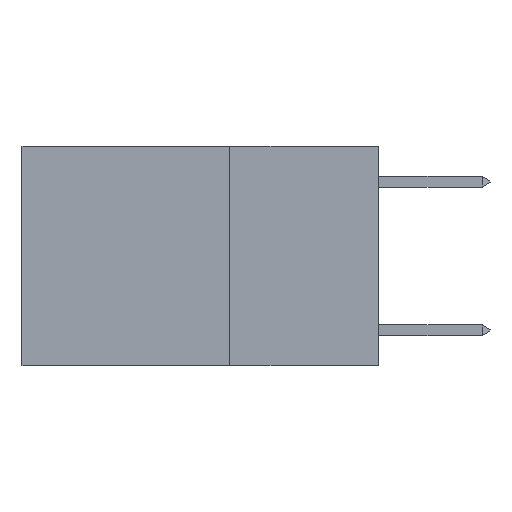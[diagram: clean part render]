
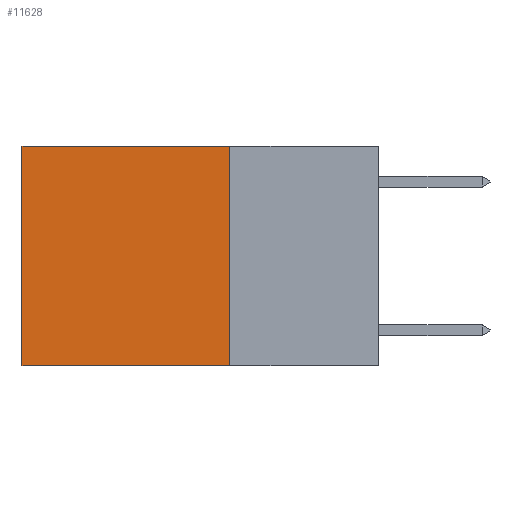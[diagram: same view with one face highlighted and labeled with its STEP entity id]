
A CAD part, left-side view. The second image highlights one B-rep face of the part: STEP entity #11628.
In plain terms, the highlighted planar face has unit normal (-1, 0, 0).
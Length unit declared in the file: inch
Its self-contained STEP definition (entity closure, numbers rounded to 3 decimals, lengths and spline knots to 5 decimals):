
#13 = CARTESIAN_POINT ( 'NONE',  ( 0.2625, 0.25, -0.37 ) ) ;
#211 = DIRECTION ( 'NONE',  ( 0., 0., -1. ) ) ;
#406 = DIRECTION ( 'NONE',  ( 1., 0., 0. ) ) ;
#1454 = DIRECTION ( 'NONE',  ( 0., 0., -1. ) ) ;
#2132 = ORIENTED_EDGE ( 'NONE', *, *, #9525, .F. ) ;
#2313 = CARTESIAN_POINT ( 'NONE',  ( 0.2625, 0.25, 0. ) ) ;
#2341 = CARTESIAN_POINT ( 'NONE',  ( 0.2625, 0.6, 0. ) ) ;
#3111 = EDGE_LOOP ( 'NONE', ( #7426, #9979, #2132, #9470 ) ) ;
#3143 = CARTESIAN_POINT ( 'NONE',  ( 0.2625, 0.25, 0. ) ) ;
#3300 = VERTEX_POINT ( 'NONE', #10219 ) ;
#3956 = LINE ( 'NONE', #13, #11379 ) ;
#4153 = LINE ( 'NONE', #3143, #11123 ) ;
#4418 = EDGE_CURVE ( 'NONE', #9586, #8267, #7765, .T. ) ;
#4705 = DIRECTION ( 'NONE',  ( 0., 0., -1. ) ) ;
#4857 = AXIS2_PLACEMENT_3D ( 'NONE', #2313, #406, #211 ) ;
#5376 = LINE ( 'NONE', #6614, #8324 ) ;
#5546 = PLANE ( 'NONE',  #4857 ) ;
#5997 = CARTESIAN_POINT ( 'NONE',  ( 0.2625, 0.6, -0.37 ) ) ;
#6614 = CARTESIAN_POINT ( 'NONE',  ( 0.2625, 0.25, 0. ) ) ;
#6640 = EDGE_CURVE ( 'NONE', #3300, #9586, #4153, .T. ) ;
#7263 = DIRECTION ( 'NONE',  ( 0., 1., 0. ) ) ;
#7426 = ORIENTED_EDGE ( 'NONE', *, *, #4418, .T. ) ;
#7758 = VECTOR ( 'NONE', #4705, 39.37008 ) ;
#7765 = LINE ( 'NONE', #11892, #7758 ) ;
#8093 = DIRECTION ( 'NONE',  ( 0., 1., 0. ) ) ;
#8267 = VERTEX_POINT ( 'NONE', #5997 ) ;
#8324 = VECTOR ( 'NONE', #1454, 39.37008 ) ;
#9436 = CARTESIAN_POINT ( 'NONE',  ( 0.2625, 0.25, -0.37 ) ) ;
#9470 = ORIENTED_EDGE ( 'NONE', *, *, #6640, .T. ) ;
#9525 = EDGE_CURVE ( 'NONE', #3300, #11783, #5376, .T. ) ;
#9586 = VERTEX_POINT ( 'NONE', #2341 ) ;
#9979 = ORIENTED_EDGE ( 'NONE', *, *, #10323, .F. ) ;
#10219 = CARTESIAN_POINT ( 'NONE',  ( 0.2625, 0.25, 0. ) ) ;
#10323 = EDGE_CURVE ( 'NONE', #11783, #8267, #3956, .T. ) ;
#11123 = VECTOR ( 'NONE', #7263, 39.37008 ) ;
#11379 = VECTOR ( 'NONE', #8093, 39.37008 ) ;
#11628 = ADVANCED_FACE ( 'NONE', ( #12808 ), #5546, .F. ) ;
#11783 = VERTEX_POINT ( 'NONE', #9436 ) ;
#11892 = CARTESIAN_POINT ( 'NONE',  ( 0.2625, 0.6, 0. ) ) ;
#12808 = FACE_OUTER_BOUND ( 'NONE', #3111, .T. ) ;
